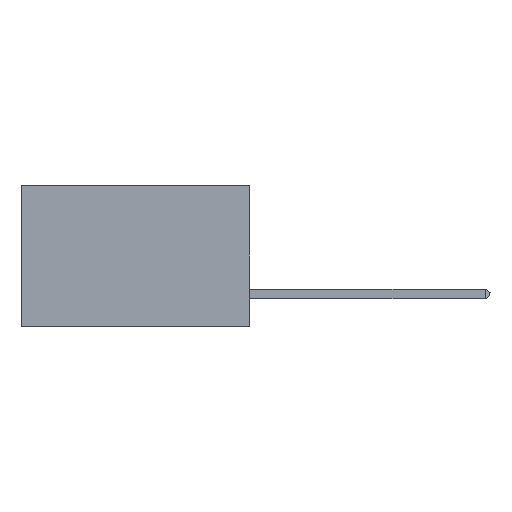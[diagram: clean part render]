
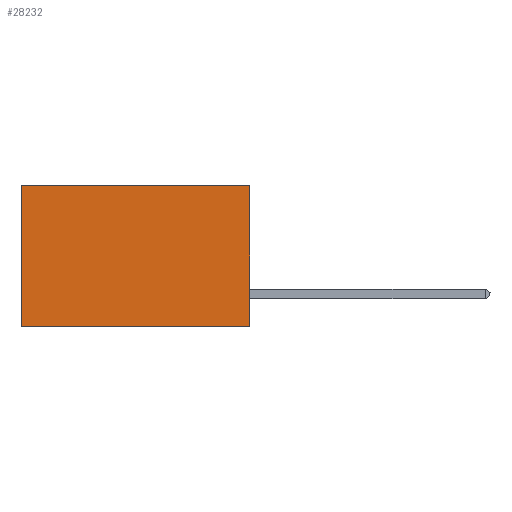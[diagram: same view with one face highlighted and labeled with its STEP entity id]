
A CAD part, left-side view. The second image highlights one B-rep face of the part: STEP entity #28232.
In plain terms, the highlighted planar face has unit normal (-1, 0, 0).
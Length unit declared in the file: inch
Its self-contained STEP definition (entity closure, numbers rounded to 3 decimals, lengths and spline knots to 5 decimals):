
#4206 = VECTOR ( 'NONE', #40833, 39.37008 ) ;
#5016 = EDGE_LOOP ( 'NONE', ( #25512, #7817, #11369, #26149 ) ) ;
#5103 = CARTESIAN_POINT ( 'NONE',  ( 0.2875, 0.6, 0. ) ) ;
#6114 = CARTESIAN_POINT ( 'NONE',  ( 0.2875, 0., 0. ) ) ;
#7817 = ORIENTED_EDGE ( 'NONE', *, *, #29275, .F. ) ;
#8024 = VERTEX_POINT ( 'NONE', #40306 ) ;
#8521 = VERTEX_POINT ( 'NONE', #32359 ) ;
#9146 = VERTEX_POINT ( 'NONE', #32650 ) ;
#11369 = ORIENTED_EDGE ( 'NONE', *, *, #37188, .F. ) ;
#11455 = CARTESIAN_POINT ( 'NONE',  ( 0.2875, 0., -0.37 ) ) ;
#12283 = DIRECTION ( 'NONE',  ( 0., 1., 0. ) ) ;
#14965 = PLANE ( 'NONE',  #30766 ) ;
#15397 = CARTESIAN_POINT ( 'NONE',  ( 0.2875, 0., 0. ) ) ;
#16636 = VECTOR ( 'NONE', #24715, 39.37008 ) ;
#18247 = DIRECTION ( 'NONE',  ( 0., 0., -1. ) ) ;
#18451 = VERTEX_POINT ( 'NONE', #23430 ) ;
#23430 = CARTESIAN_POINT ( 'NONE',  ( 0.2875, 0.6, 0. ) ) ;
#24715 = DIRECTION ( 'NONE',  ( 0., 0., -1. ) ) ;
#25512 = ORIENTED_EDGE ( 'NONE', *, *, #28198, .T. ) ;
#26149 = ORIENTED_EDGE ( 'NONE', *, *, #39725, .T. ) ;
#27196 = LINE ( 'NONE', #27473, #32371 ) ;
#27473 = CARTESIAN_POINT ( 'NONE',  ( 0.2875, 0., 0. ) ) ;
#28198 = EDGE_CURVE ( 'NONE', #18451, #8024, #39738, .T. ) ;
#28232 = ADVANCED_FACE ( 'NONE', ( #38714 ), #14965, .F. ) ;
#29275 = EDGE_CURVE ( 'NONE', #9146, #8024, #30932, .T. ) ;
#30766 = AXIS2_PLACEMENT_3D ( 'NONE', #15397, #31904, #18247 ) ;
#30791 = DIRECTION ( 'NONE',  ( 0., 0., -1. ) ) ;
#30932 = LINE ( 'NONE', #11455, #4206 ) ;
#31904 = DIRECTION ( 'NONE',  ( 1., 0., 0. ) ) ;
#32359 = CARTESIAN_POINT ( 'NONE',  ( 0.2875, 0., 0. ) ) ;
#32371 = VECTOR ( 'NONE', #30791, 39.37008 ) ;
#32650 = CARTESIAN_POINT ( 'NONE',  ( 0.2875, 0., -0.37 ) ) ;
#35807 = LINE ( 'NONE', #6114, #38862 ) ;
#37188 = EDGE_CURVE ( 'NONE', #8521, #9146, #27196, .T. ) ;
#38714 = FACE_OUTER_BOUND ( 'NONE', #5016, .T. ) ;
#38862 = VECTOR ( 'NONE', #12283, 39.37008 ) ;
#39725 = EDGE_CURVE ( 'NONE', #8521, #18451, #35807, .T. ) ;
#39738 = LINE ( 'NONE', #5103, #16636 ) ;
#40306 = CARTESIAN_POINT ( 'NONE',  ( 0.2875, 0.6, -0.37 ) ) ;
#40833 = DIRECTION ( 'NONE',  ( 0., 1., 0. ) ) ;
